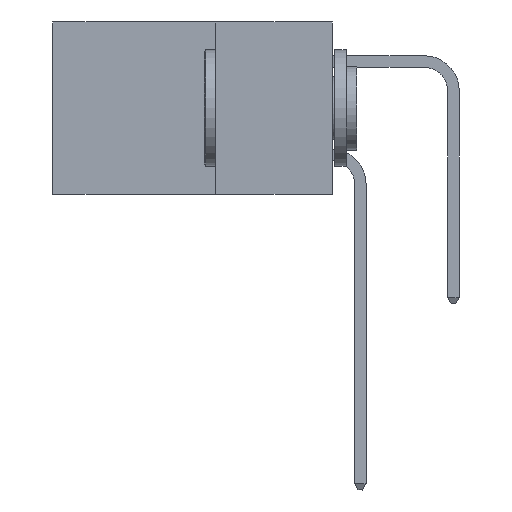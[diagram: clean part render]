
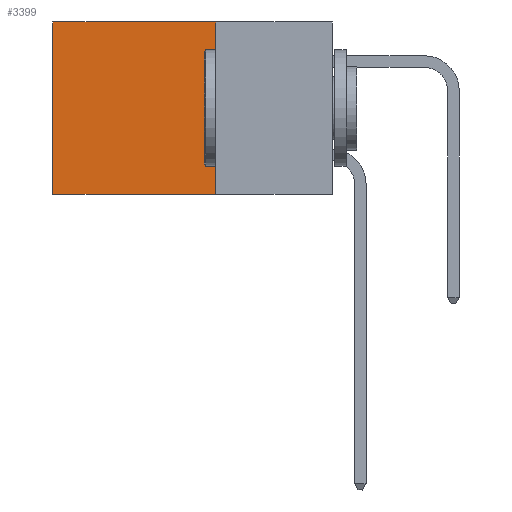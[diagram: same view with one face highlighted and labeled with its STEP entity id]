
A CAD part, left-side view. The second image highlights one B-rep face of the part: STEP entity #3399.
In plain terms, the highlighted planar face has unit normal (-1, 0, 0).
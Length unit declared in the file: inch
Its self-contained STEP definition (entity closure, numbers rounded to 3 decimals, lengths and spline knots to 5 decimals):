
#163 = VERTEX_POINT ( 'NONE', #18152 ) ;
#193 = VECTOR ( 'NONE', #18890, 39.37008 ) ;
#2395 = VECTOR ( 'NONE', #29202, 39.37008 ) ;
#2821 = VERTEX_POINT ( 'NONE', #31093 ) ;
#3199 = CARTESIAN_POINT ( 'NONE',  ( 0.298, 0.25, 0. ) ) ;
#3399 = ADVANCED_FACE ( 'NONE', ( #31067 ), #10729, .F. ) ;
#4076 = DIRECTION ( 'NONE',  ( 0., 1., 0. ) ) ;
#4087 = VERTEX_POINT ( 'NONE', #30909 ) ;
#4414 = LINE ( 'NONE', #26536, #193 ) ;
#5635 = CARTESIAN_POINT ( 'NONE',  ( 0.298, 0.25, 0. ) ) ;
#7142 = EDGE_CURVE ( 'NONE', #23200, #2821, #11624, .T. ) ;
#8205 = VECTOR ( 'NONE', #26546, 39.37008 ) ;
#8218 = EDGE_CURVE ( 'NONE', #2821, #163, #19373, .T. ) ;
#9430 = CARTESIAN_POINT ( 'NONE',  ( 0.298, 0.6, 0. ) ) ;
#10729 = PLANE ( 'NONE',  #11439 ) ;
#11235 = EDGE_CURVE ( 'NONE', #4087, #163, #26004, .T. ) ;
#11439 = AXIS2_PLACEMENT_3D ( 'NONE', #3199, #30552, #25485 ) ;
#11484 = CARTESIAN_POINT ( 'NONE',  ( 0.298, 0.25, -0.37 ) ) ;
#11624 = LINE ( 'NONE', #14474, #2395 ) ;
#12934 = ORIENTED_EDGE ( 'NONE', *, *, #27138, .F. ) ;
#12982 = VECTOR ( 'NONE', #4076, 39.37008 ) ;
#14474 = CARTESIAN_POINT ( 'NONE',  ( 0.298, 0.25, 0. ) ) ;
#16987 = ORIENTED_EDGE ( 'NONE', *, *, #11235, .F. ) ;
#18152 = CARTESIAN_POINT ( 'NONE',  ( 0.298, 0.6, -0.37 ) ) ;
#18890 = DIRECTION ( 'NONE',  ( 0., 0., -1. ) ) ;
#19373 = LINE ( 'NONE', #9430, #8205 ) ;
#21517 = EDGE_LOOP ( 'NONE', ( #21760, #16987, #12934, #28810 ) ) ;
#21760 = ORIENTED_EDGE ( 'NONE', *, *, #8218, .T. ) ;
#23200 = VERTEX_POINT ( 'NONE', #5635 ) ;
#25485 = DIRECTION ( 'NONE',  ( 0., 0., -1. ) ) ;
#26004 = LINE ( 'NONE', #11484, #12982 ) ;
#26536 = CARTESIAN_POINT ( 'NONE',  ( 0.298, 0.25, 0. ) ) ;
#26546 = DIRECTION ( 'NONE',  ( 0., 0., -1. ) ) ;
#27138 = EDGE_CURVE ( 'NONE', #23200, #4087, #4414, .T. ) ;
#28810 = ORIENTED_EDGE ( 'NONE', *, *, #7142, .T. ) ;
#29202 = DIRECTION ( 'NONE',  ( 0., 1., 0. ) ) ;
#30552 = DIRECTION ( 'NONE',  ( 1., 0., 0. ) ) ;
#30909 = CARTESIAN_POINT ( 'NONE',  ( 0.298, 0.25, -0.37 ) ) ;
#31067 = FACE_OUTER_BOUND ( 'NONE', #21517, .T. ) ;
#31093 = CARTESIAN_POINT ( 'NONE',  ( 0.298, 0.6, 0. ) ) ;
